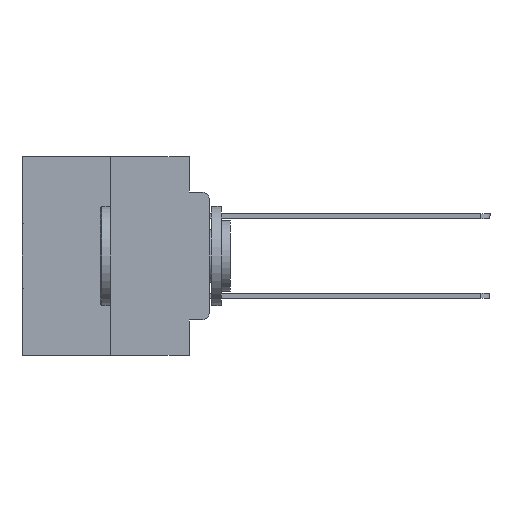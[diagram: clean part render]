
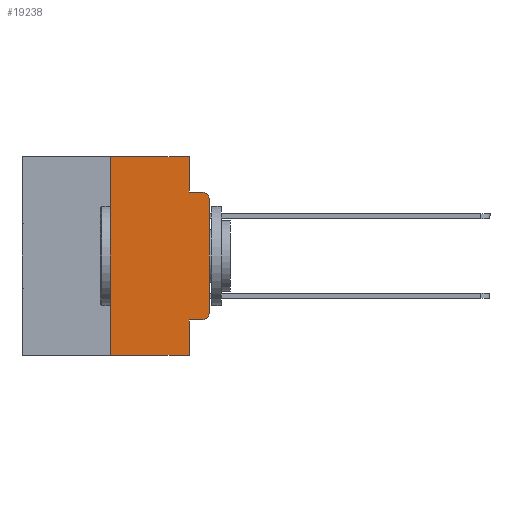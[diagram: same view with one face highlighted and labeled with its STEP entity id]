
A CAD part, left-side view. The second image highlights one B-rep face of the part: STEP entity #19238.
In plain terms, the highlighted planar face has unit normal (-1, 0, 0).
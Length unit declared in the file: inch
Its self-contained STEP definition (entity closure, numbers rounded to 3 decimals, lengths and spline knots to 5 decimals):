
#471 = VECTOR ( 'NONE', #19053, 39.37008 ) ;
#1732 = EDGE_LOOP ( 'NONE', ( #29106, #25506, #25260, #25141, #24856, #24743, #24092, #23763, #23649, #23416 ) ) ;
#1761 = VECTOR ( 'NONE', #8623, 39.37008 ) ;
#2214 = AXIS2_PLACEMENT_3D ( 'NONE', #4289, #20999, #6742 ) ;
#2498 = VECTOR ( 'NONE', #24829, 39.37008 ) ;
#3273 = LINE ( 'NONE', #10578, #2498 ) ;
#3600 = CARTESIAN_POINT ( 'NONE',  ( 0., 0., -0.3915 ) ) ;
#3893 = VERTEX_POINT ( 'NONE', #15926 ) ;
#4289 = CARTESIAN_POINT ( 'NONE',  ( 0., 0.473, 0. ) ) ;
#4945 = EDGE_CURVE ( 'NONE', #21288, #22933, #3273, .T. ) ;
#5084 = CIRCLE ( 'NONE', #14348, 0.02 ) ;
#5762 = CARTESIAN_POINT ( 'NONE',  ( 0., 0.25, -0.5 ) ) ;
#6742 = DIRECTION ( 'NONE',  ( 0., 0., -1. ) ) ;
#7006 = VECTOR ( 'NONE', #21779, 39.37008 ) ;
#7048 = VECTOR ( 'NONE', #7671, 39.37008 ) ;
#7559 = VERTEX_POINT ( 'NONE', #5762 ) ;
#7593 = EDGE_CURVE ( 'NONE', #15243, #20917, #5084, .T. ) ;
#7632 = CARTESIAN_POINT ( 'NONE',  ( 0., 0.25, 0. ) ) ;
#7671 = DIRECTION ( 'NONE',  ( 0., -1., 0. ) ) ;
#8200 = DIRECTION ( 'NONE',  ( 0., -1., 0. ) ) ;
#8560 = LINE ( 'NONE', #27255, #20443 ) ;
#8623 = DIRECTION ( 'NONE',  ( 0., 0., 1. ) ) ;
#9191 = CIRCLE ( 'NONE', #12201, 0.02 ) ;
#9379 = CARTESIAN_POINT ( 'NONE',  ( 0., 0.02, -0.0885 ) ) ;
#10031 = DIRECTION ( 'NONE',  ( -1., 0., 0. ) ) ;
#10058 = VERTEX_POINT ( 'NONE', #10813 ) ;
#10578 = CARTESIAN_POINT ( 'NONE',  ( 0., 0.473, 0. ) ) ;
#10813 = CARTESIAN_POINT ( 'NONE',  ( 0., 0.051, -0.5 ) ) ;
#11034 = CARTESIAN_POINT ( 'NONE',  ( 0., 0., 0. ) ) ;
#11308 = LINE ( 'NONE', #11034, #1761 ) ;
#11954 = LINE ( 'NONE', #23868, #471 ) ;
#12088 = EDGE_CURVE ( 'NONE', #7559, #21288, #12868, .T. ) ;
#12201 = AXIS2_PLACEMENT_3D ( 'NONE', #24283, #10031, #26669 ) ;
#12868 = LINE ( 'NONE', #24786, #24799 ) ;
#12904 = DIRECTION ( 'NONE',  ( 0., 0., 1. ) ) ;
#13075 = DIRECTION ( 'NONE',  ( -1., 0., 0. ) ) ;
#14250 = VERTEX_POINT ( 'NONE', #9379 ) ;
#14348 = AXIS2_PLACEMENT_3D ( 'NONE', #27344, #13075, #29709 ) ;
#14685 = EDGE_CURVE ( 'NONE', #20917, #18328, #11308, .T. ) ;
#15243 = VERTEX_POINT ( 'NONE', #20433 ) ;
#15926 = CARTESIAN_POINT ( 'NONE',  ( 0., 0.051, -0.0885 ) ) ;
#16030 = PLANE ( 'NONE',  #2214 ) ;
#16318 = EDGE_CURVE ( 'NONE', #7559, #10058, #18949, .T. ) ;
#16615 = LINE ( 'NONE', #29956, #21436 ) ;
#17386 = EDGE_CURVE ( 'NONE', #25744, #15243, #11954, .T. ) ;
#18328 = VERTEX_POINT ( 'NONE', #24720 ) ;
#18884 = CARTESIAN_POINT ( 'NONE',  ( 0., 0.051, -0.4115 ) ) ;
#18949 = LINE ( 'NONE', #21902, #7048 ) ;
#19053 = DIRECTION ( 'NONE',  ( 0., -1., 0. ) ) ;
#19238 = ADVANCED_FACE ( 'NONE', ( #25249 ), #16030, .F. ) ;
#19398 = CARTESIAN_POINT ( 'NONE',  ( 0., 0.051, 0. ) ) ;
#20091 = EDGE_CURVE ( 'NONE', #18328, #14250, #9191, .T. ) ;
#20433 = CARTESIAN_POINT ( 'NONE',  ( 0., 0.02, -0.4115 ) ) ;
#20443 = VECTOR ( 'NONE', #8200, 39.37008 ) ;
#20917 = VERTEX_POINT ( 'NONE', #3600 ) ;
#20999 = DIRECTION ( 'NONE',  ( 1., 0., 0. ) ) ;
#21288 = VERTEX_POINT ( 'NONE', #7632 ) ;
#21436 = VECTOR ( 'NONE', #22887, 39.37008 ) ;
#21779 = DIRECTION ( 'NONE',  ( 0., 0., -1. ) ) ;
#21902 = CARTESIAN_POINT ( 'NONE',  ( 0., 0.473, -0.5 ) ) ;
#22887 = DIRECTION ( 'NONE',  ( 0., 0., -1. ) ) ;
#22933 = VERTEX_POINT ( 'NONE', #25980 ) ;
#23416 = ORIENTED_EDGE ( 'NONE', *, *, #7593, .T. ) ;
#23606 = EDGE_CURVE ( 'NONE', #25744, #10058, #16615, .T. ) ;
#23649 = ORIENTED_EDGE ( 'NONE', *, *, #17386, .T. ) ;
#23763 = ORIENTED_EDGE ( 'NONE', *, *, #23606, .F. ) ;
#23868 = CARTESIAN_POINT ( 'NONE',  ( 0., 0.051, -0.4115 ) ) ;
#24092 = ORIENTED_EDGE ( 'NONE', *, *, #16318, .T. ) ;
#24283 = CARTESIAN_POINT ( 'NONE',  ( 0., 0.02, -0.1085 ) ) ;
#24720 = CARTESIAN_POINT ( 'NONE',  ( 0., 0., -0.1085 ) ) ;
#24743 = ORIENTED_EDGE ( 'NONE', *, *, #12088, .F. ) ;
#24786 = CARTESIAN_POINT ( 'NONE',  ( 0., 0.25, 0. ) ) ;
#24799 = VECTOR ( 'NONE', #12904, 39.37008 ) ;
#24829 = DIRECTION ( 'NONE',  ( 0., -1., 0. ) ) ;
#24856 = ORIENTED_EDGE ( 'NONE', *, *, #4945, .F. ) ;
#25141 = ORIENTED_EDGE ( 'NONE', *, *, #30013, .F. ) ;
#25249 = FACE_OUTER_BOUND ( 'NONE', #1732, .T. ) ;
#25260 = ORIENTED_EDGE ( 'NONE', *, *, #27680, .F. ) ;
#25506 = ORIENTED_EDGE ( 'NONE', *, *, #20091, .T. ) ;
#25744 = VERTEX_POINT ( 'NONE', #18884 ) ;
#25980 = CARTESIAN_POINT ( 'NONE',  ( 0., 0.051, 0. ) ) ;
#26010 = LINE ( 'NONE', #19398, #7006 ) ;
#26669 = DIRECTION ( 'NONE',  ( 0., 0., -1. ) ) ;
#27255 = CARTESIAN_POINT ( 'NONE',  ( 0., 0.051, -0.0885 ) ) ;
#27344 = CARTESIAN_POINT ( 'NONE',  ( 0., 0.02, -0.3915 ) ) ;
#27680 = EDGE_CURVE ( 'NONE', #3893, #14250, #8560, .T. ) ;
#29106 = ORIENTED_EDGE ( 'NONE', *, *, #14685, .T. ) ;
#29709 = DIRECTION ( 'NONE',  ( 0., 0., -1. ) ) ;
#29956 = CARTESIAN_POINT ( 'NONE',  ( 0., 0.051, 0. ) ) ;
#30013 = EDGE_CURVE ( 'NONE', #22933, #3893, #26010, .T. ) ;
